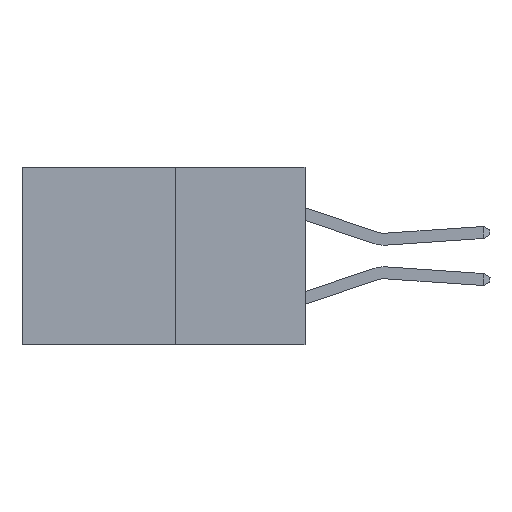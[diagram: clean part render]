
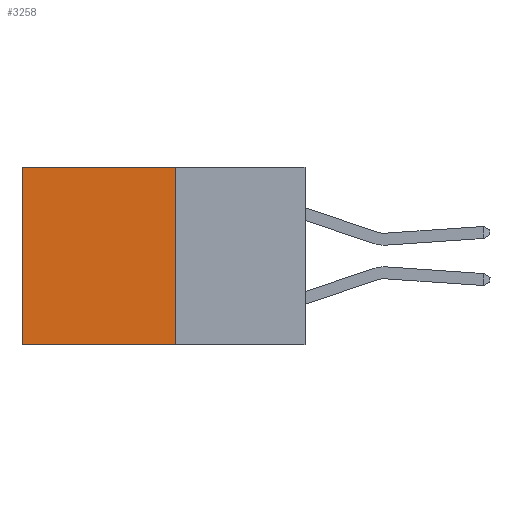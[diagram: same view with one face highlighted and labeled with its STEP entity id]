
A CAD part, left-side view. The second image highlights one B-rep face of the part: STEP entity #3258.
In plain terms, the highlighted planar face has unit normal (-1, 0, 0).
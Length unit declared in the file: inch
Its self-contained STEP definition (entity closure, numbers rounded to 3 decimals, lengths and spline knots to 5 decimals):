
#498 = ORIENTED_EDGE ( 'NONE', *, *, #26733, .T. ) ;
#1823 = FACE_OUTER_BOUND ( 'NONE', #13341, .T. ) ;
#2619 = VECTOR ( 'NONE', #27193, 39.37008 ) ;
#3258 = ADVANCED_FACE ( 'NONE', ( #1823 ), #14881, .F. ) ;
#3745 = CARTESIAN_POINT ( 'NONE',  ( 0.277, 0.59, 0. ) ) ;
#4465 = CARTESIAN_POINT ( 'NONE',  ( 0.277, 0.59, -0.37 ) ) ;
#5742 = ORIENTED_EDGE ( 'NONE', *, *, #7591, .F. ) ;
#6632 = VECTOR ( 'NONE', #16495, 39.37008 ) ;
#6692 = ORIENTED_EDGE ( 'NONE', *, *, #27725, .F. ) ;
#7059 = VERTEX_POINT ( 'NONE', #13765 ) ;
#7591 = EDGE_CURVE ( 'NONE', #12674, #7059, #14713, .T. ) ;
#7648 = CARTESIAN_POINT ( 'NONE',  ( 0.277, 0.27, 0. ) ) ;
#8688 = VECTOR ( 'NONE', #14246, 39.37008 ) ;
#8957 = VERTEX_POINT ( 'NONE', #4465 ) ;
#9102 = VECTOR ( 'NONE', #22200, 39.37008 ) ;
#9807 = LINE ( 'NONE', #19975, #9102 ) ;
#11214 = VERTEX_POINT ( 'NONE', #3745 ) ;
#11589 = AXIS2_PLACEMENT_3D ( 'NONE', #16987, #22678, #24238 ) ;
#11991 = CARTESIAN_POINT ( 'NONE',  ( 0.277, 0.27, 0. ) ) ;
#12674 = VERTEX_POINT ( 'NONE', #7648 ) ;
#13341 = EDGE_LOOP ( 'NONE', ( #498, #6692, #5742, #16690 ) ) ;
#13359 = LINE ( 'NONE', #18767, #6632 ) ;
#13765 = CARTESIAN_POINT ( 'NONE',  ( 0.277, 0.27, -0.37 ) ) ;
#14246 = DIRECTION ( 'NONE',  ( 0., 1., 0. ) ) ;
#14713 = LINE ( 'NONE', #27388, #2619 ) ;
#14881 = PLANE ( 'NONE',  #11589 ) ;
#16495 = DIRECTION ( 'NONE',  ( 0., 0., -1. ) ) ;
#16690 = ORIENTED_EDGE ( 'NONE', *, *, #28356, .T. ) ;
#16987 = CARTESIAN_POINT ( 'NONE',  ( 0.277, 0.27, -0.37 ) ) ;
#18767 = CARTESIAN_POINT ( 'NONE',  ( 0.277, 0.59, -0.37 ) ) ;
#19975 = CARTESIAN_POINT ( 'NONE',  ( 0.277, 0.27, -0.37 ) ) ;
#22200 = DIRECTION ( 'NONE',  ( 0., 1., 0. ) ) ;
#22678 = DIRECTION ( 'NONE',  ( 1., 0., 0. ) ) ;
#24238 = DIRECTION ( 'NONE',  ( 0., 0., -1. ) ) ;
#26519 = LINE ( 'NONE', #11991, #8688 ) ;
#26733 = EDGE_CURVE ( 'NONE', #11214, #8957, #13359, .T. ) ;
#27193 = DIRECTION ( 'NONE',  ( 0., 0., -1. ) ) ;
#27388 = CARTESIAN_POINT ( 'NONE',  ( 0.277, 0.27, -0.37 ) ) ;
#27725 = EDGE_CURVE ( 'NONE', #7059, #8957, #9807, .T. ) ;
#28356 = EDGE_CURVE ( 'NONE', #12674, #11214, #26519, .T. ) ;
